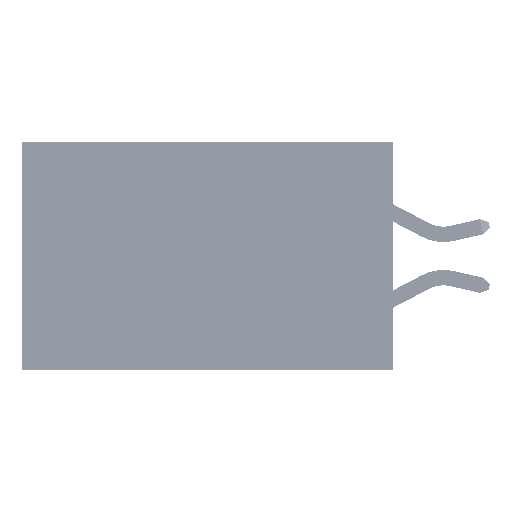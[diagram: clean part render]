
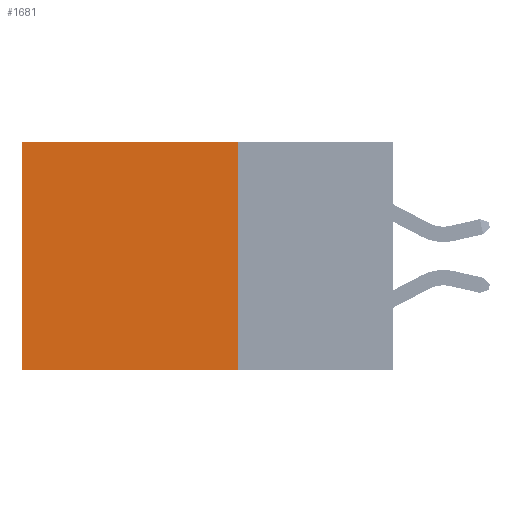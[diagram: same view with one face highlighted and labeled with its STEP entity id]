
A CAD part, left-side view. The second image highlights one B-rep face of the part: STEP entity #1681.
In plain terms, the highlighted planar face has unit normal (-1, 0, 0).
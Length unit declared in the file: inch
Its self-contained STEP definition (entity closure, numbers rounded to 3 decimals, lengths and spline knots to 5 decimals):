
#340 = EDGE_CURVE ( 'NONE', #41531, #44892, #3510, .T. ) ;
#1681 = ADVANCED_FACE ( 'NONE', ( #27110 ), #39398, .F. ) ;
#1793 = LINE ( 'NONE', #2040, #39090 ) ;
#2040 = CARTESIAN_POINT ( 'NONE',  ( 0.2875, 0.25, 0. ) ) ;
#2160 = CARTESIAN_POINT ( 'NONE',  ( 0.2875, 0.25, 0. ) ) ;
#3510 = LINE ( 'NONE', #34200, #33910 ) ;
#3808 = ORIENTED_EDGE ( 'NONE', *, *, #27602, .F. ) ;
#8897 = VECTOR ( 'NONE', #30051, 39.37008 ) ;
#11748 = DIRECTION ( 'NONE',  ( 0., 0., -1. ) ) ;
#15062 = DIRECTION ( 'NONE',  ( 0., 1., 0. ) ) ;
#15998 = EDGE_LOOP ( 'NONE', ( #26929, #3808, #25680, #35349 ) ) ;
#18005 = AXIS2_PLACEMENT_3D ( 'NONE', #19692, #20185, #11748 ) ;
#19692 = CARTESIAN_POINT ( 'NONE',  ( 0.2875, 0.25, 0. ) ) ;
#20182 = VERTEX_POINT ( 'NONE', #43409 ) ;
#20185 = DIRECTION ( 'NONE',  ( 1., 0., 0. ) ) ;
#25680 = ORIENTED_EDGE ( 'NONE', *, *, #340, .F. ) ;
#26929 = ORIENTED_EDGE ( 'NONE', *, *, #31010, .T. ) ;
#27110 = FACE_OUTER_BOUND ( 'NONE', #15998, .T. ) ;
#27602 = EDGE_CURVE ( 'NONE', #44892, #28870, #38876, .T. ) ;
#28870 = VERTEX_POINT ( 'NONE', #33729 ) ;
#29296 = CARTESIAN_POINT ( 'NONE',  ( 0.2875, 0.6, 0. ) ) ;
#30009 = EDGE_CURVE ( 'NONE', #41531, #20182, #1793, .T. ) ;
#30051 = DIRECTION ( 'NONE',  ( 0., 0., -1. ) ) ;
#31010 = EDGE_CURVE ( 'NONE', #20182, #28870, #49516, .T. ) ;
#31186 = CARTESIAN_POINT ( 'NONE',  ( 0.2875, 0.25, -0.37 ) ) ;
#33729 = CARTESIAN_POINT ( 'NONE',  ( 0.2875, 0.6, -0.37 ) ) ;
#33910 = VECTOR ( 'NONE', #38305, 39.37008 ) ;
#34200 = CARTESIAN_POINT ( 'NONE',  ( 0.2875, 0.25, 0. ) ) ;
#35349 = ORIENTED_EDGE ( 'NONE', *, *, #30009, .T. ) ;
#37093 = DIRECTION ( 'NONE',  ( 0., 1., 0. ) ) ;
#38305 = DIRECTION ( 'NONE',  ( 0., 0., -1. ) ) ;
#38876 = LINE ( 'NONE', #31186, #40612 ) ;
#39090 = VECTOR ( 'NONE', #37093, 39.37008 ) ;
#39398 = PLANE ( 'NONE',  #18005 ) ;
#40612 = VECTOR ( 'NONE', #15062, 39.37008 ) ;
#41531 = VERTEX_POINT ( 'NONE', #2160 ) ;
#42539 = CARTESIAN_POINT ( 'NONE',  ( 0.2875, 0.25, -0.37 ) ) ;
#43409 = CARTESIAN_POINT ( 'NONE',  ( 0.2875, 0.6, 0. ) ) ;
#44892 = VERTEX_POINT ( 'NONE', #42539 ) ;
#49516 = LINE ( 'NONE', #29296, #8897 ) ;
